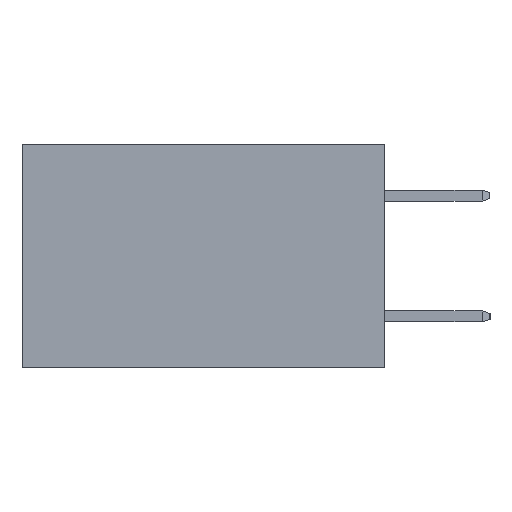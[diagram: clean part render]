
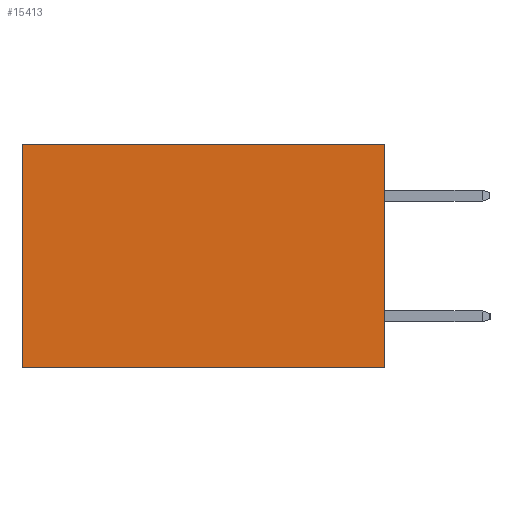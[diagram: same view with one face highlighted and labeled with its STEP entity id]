
A CAD part, left-side view. The second image highlights one B-rep face of the part: STEP entity #15413.
In plain terms, the highlighted planar face has unit normal (-1, 0, 0).
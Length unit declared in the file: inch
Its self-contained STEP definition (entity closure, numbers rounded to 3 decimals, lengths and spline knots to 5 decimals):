
#1008 = LINE ( 'NONE', #4208, #4584 ) ;
#1320 = EDGE_LOOP ( 'NONE', ( #8480, #16479, #18533, #11384 ) ) ;
#1806 = DIRECTION ( 'NONE',  ( 0., 1., 0. ) ) ;
#2339 = CARTESIAN_POINT ( 'NONE',  ( 0.2615, 0.6, 0. ) ) ;
#2583 = FACE_OUTER_BOUND ( 'NONE', #1320, .T. ) ;
#3001 = PLANE ( 'NONE',  #16488 ) ;
#3249 = LINE ( 'NONE', #12365, #10650 ) ;
#3263 = VERTEX_POINT ( 'NONE', #11214 ) ;
#3872 = VECTOR ( 'NONE', #1806, 39.37008 ) ;
#4208 = CARTESIAN_POINT ( 'NONE',  ( 0.2615, 0.6, -0.37 ) ) ;
#4495 = DIRECTION ( 'NONE',  ( 0., 0., -1. ) ) ;
#4584 = VECTOR ( 'NONE', #16018, 39.37008 ) ;
#4886 = EDGE_CURVE ( 'NONE', #3263, #5429, #3249, .T. ) ;
#5429 = VERTEX_POINT ( 'NONE', #16016 ) ;
#5834 = DIRECTION ( 'NONE',  ( 0., 0., -1. ) ) ;
#8480 = ORIENTED_EDGE ( 'NONE', *, *, #17619, .T. ) ;
#9767 = CARTESIAN_POINT ( 'NONE',  ( 0.2615, 0., 0. ) ) ;
#10204 = CARTESIAN_POINT ( 'NONE',  ( 0.2615, 0., -0.37 ) ) ;
#10619 = VERTEX_POINT ( 'NONE', #2339 ) ;
#10650 = VECTOR ( 'NONE', #11574, 39.37008 ) ;
#10714 = CARTESIAN_POINT ( 'NONE',  ( 0.2615, 0., 0. ) ) ;
#11214 = CARTESIAN_POINT ( 'NONE',  ( 0.2615, 0., -0.37 ) ) ;
#11384 = ORIENTED_EDGE ( 'NONE', *, *, #18993, .T. ) ;
#11390 = VERTEX_POINT ( 'NONE', #9767 ) ;
#11574 = DIRECTION ( 'NONE',  ( 0., 1., 0. ) ) ;
#12141 = EDGE_CURVE ( 'NONE', #11390, #3263, #12446, .T. ) ;
#12365 = CARTESIAN_POINT ( 'NONE',  ( 0.2615, 0., -0.37 ) ) ;
#12446 = LINE ( 'NONE', #10204, #15884 ) ;
#13374 = DIRECTION ( 'NONE',  ( 1., 0., 0. ) ) ;
#15413 = ADVANCED_FACE ( 'NONE', ( #2583 ), #3001, .F. ) ;
#15884 = VECTOR ( 'NONE', #5834, 39.37008 ) ;
#16016 = CARTESIAN_POINT ( 'NONE',  ( 0.2615, 0.6, -0.37 ) ) ;
#16018 = DIRECTION ( 'NONE',  ( 0., 0., -1. ) ) ;
#16479 = ORIENTED_EDGE ( 'NONE', *, *, #4886, .F. ) ;
#16488 = AXIS2_PLACEMENT_3D ( 'NONE', #19063, #13374, #4495 ) ;
#17619 = EDGE_CURVE ( 'NONE', #10619, #5429, #1008, .T. ) ;
#18533 = ORIENTED_EDGE ( 'NONE', *, *, #12141, .F. ) ;
#18965 = LINE ( 'NONE', #10714, #3872 ) ;
#18993 = EDGE_CURVE ( 'NONE', #11390, #10619, #18965, .T. ) ;
#19063 = CARTESIAN_POINT ( 'NONE',  ( 0.2615, 0., -0.37 ) ) ;
